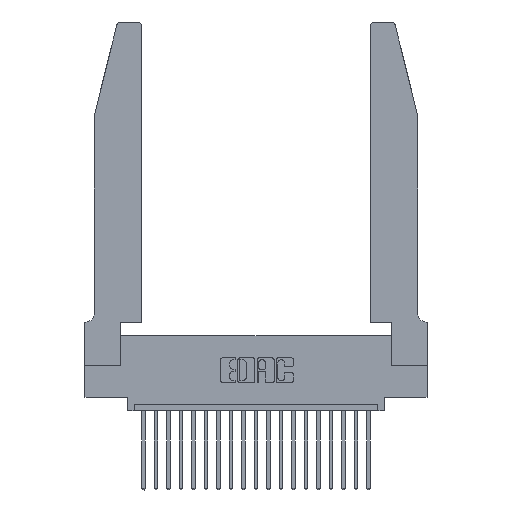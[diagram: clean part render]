
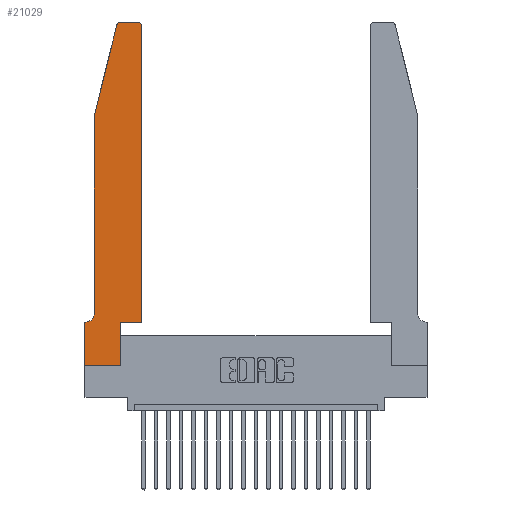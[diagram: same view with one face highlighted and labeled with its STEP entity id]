
A CAD part, top view. The second image highlights one B-rep face of the part: STEP entity #21029.
In plain terms, the highlighted planar face has unit normal (0, 0, 1).
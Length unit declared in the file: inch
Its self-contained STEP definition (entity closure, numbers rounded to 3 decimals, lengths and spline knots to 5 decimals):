
#202 = ORIENTED_EDGE ( 'NONE', *, *, #20439, .T. ) ;
#475 = FACE_OUTER_BOUND ( 'NONE', #21155, .T. ) ;
#745 = VECTOR ( 'NONE', #18518, 39.37008 ) ;
#861 = VECTOR ( 'NONE', #21753, 39.37008 ) ;
#864 = CARTESIAN_POINT ( 'NONE',  ( 0.2865, 0.35, 0.37 ) ) ;
#910 = CIRCLE ( 'NONE', #21484, 0.03 ) ;
#933 = CARTESIAN_POINT ( 'NONE',  ( 0., 0.35, 0.37 ) ) ;
#1227 = DIRECTION ( 'NONE',  ( 0., -1., 0. ) ) ;
#1330 = CARTESIAN_POINT ( 'NONE',  ( 0.2865, 0.35, 0.37 ) ) ;
#1549 = LINE ( 'NONE', #8775, #1835 ) ;
#1553 = EDGE_CURVE ( 'NONE', #18526, #16632, #6762, .T. ) ;
#1835 = VECTOR ( 'NONE', #8693, 39.37008 ) ;
#2358 = DIRECTION ( 'NONE',  ( -1., 0., 0. ) ) ;
#2425 = CIRCLE ( 'NONE', #20134, 0.07 ) ;
#2496 = DIRECTION ( 'NONE',  ( 0., 0., 1. ) ) ;
#2521 = ORIENTED_EDGE ( 'NONE', *, *, #2950, .T. ) ;
#2777 = VECTOR ( 'NONE', #1227, 39.37008 ) ;
#2950 = EDGE_CURVE ( 'NONE', #14759, #15121, #18261, .T. ) ;
#2978 = CARTESIAN_POINT ( 'NONE',  ( 0.0755, 2., 0.37 ) ) ;
#3802 = VECTOR ( 'NONE', #17745, 39.37008 ) ;
#3931 = VERTEX_POINT ( 'NONE', #5555 ) ;
#4231 = EDGE_CURVE ( 'NONE', #15005, #18241, #13648, .T. ) ;
#4685 = PLANE ( 'NONE',  #15133 ) ;
#5212 = DIRECTION ( 'NONE',  ( -1., 0., 0. ) ) ;
#5555 = CARTESIAN_POINT ( 'NONE',  ( 0.2865, 0., 0.37 ) ) ;
#5576 = CARTESIAN_POINT ( 'NONE',  ( 0.4505, 0.35, 0.37 ) ) ;
#5680 = EDGE_CURVE ( 'NONE', #15121, #8326, #12274, .T. ) ;
#6691 = AXIS2_PLACEMENT_3D ( 'NONE', #21542, #2496, #19594 ) ;
#6755 = VERTEX_POINT ( 'NONE', #10469 ) ;
#6762 = LINE ( 'NONE', #5576, #3802 ) ;
#6979 = ORIENTED_EDGE ( 'NONE', *, *, #16022, .T. ) ;
#7459 = DIRECTION ( 'NONE',  ( 0., 0., 1. ) ) ;
#7564 = LINE ( 'NONE', #1330, #10790 ) ;
#8105 = CARTESIAN_POINT ( 'NONE',  ( 0.4505, 0.35, 0.37 ) ) ;
#8278 = EDGE_CURVE ( 'NONE', #6755, #16567, #19460, .T. ) ;
#8314 = CARTESIAN_POINT ( 'NONE',  ( 0.0755, 2., 0.37 ) ) ;
#8326 = VERTEX_POINT ( 'NONE', #18783 ) ;
#8382 = DIRECTION ( 'NONE',  ( 0., 1., 0. ) ) ;
#8669 = CARTESIAN_POINT ( 'NONE',  ( 0., 0., 0.37 ) ) ;
#8693 = DIRECTION ( 'NONE',  ( -1., 0., 0. ) ) ;
#8696 = CARTESIAN_POINT ( 'NONE',  ( 0.0055, 0.42, 0.37 ) ) ;
#8775 = CARTESIAN_POINT ( 'NONE',  ( 0.2605, 2.75, 0.37 ) ) ;
#9259 = ORIENTED_EDGE ( 'NONE', *, *, #21108, .T. ) ;
#9622 = EDGE_CURVE ( 'NONE', #16632, #15005, #14655, .T. ) ;
#9852 = ORIENTED_EDGE ( 'NONE', *, *, #13249, .T. ) ;
#9885 = DIRECTION ( 'NONE',  ( 0., 0., 1. ) ) ;
#10398 = DIRECTION ( 'NONE',  ( 1., 0., 0. ) ) ;
#10469 = CARTESIAN_POINT ( 'NONE',  ( 0.0755, 2., 0.37 ) ) ;
#10790 = VECTOR ( 'NONE', #8382, 39.37008 ) ;
#11171 = CARTESIAN_POINT ( 'NONE',  ( 0., 0., 0.37 ) ) ;
#11232 = VECTOR ( 'NONE', #10398, 39.37008 ) ;
#11288 = ORIENTED_EDGE ( 'NONE', *, *, #1553, .T. ) ;
#12167 = DIRECTION ( 'NONE',  ( 0., 0., -1. ) ) ;
#12274 = LINE ( 'NONE', #11171, #14960 ) ;
#12591 = ORIENTED_EDGE ( 'NONE', *, *, #5680, .T. ) ;
#12627 = DIRECTION ( 'NONE',  ( 1., 0., 0. ) ) ;
#12697 = CARTESIAN_POINT ( 'NONE',  ( 0.284, 2.72, 0.37 ) ) ;
#13249 = EDGE_CURVE ( 'NONE', #8326, #3931, #22232, .T. ) ;
#13416 = CARTESIAN_POINT ( 'NONE',  ( 0.4505, 2.72, 0.37 ) ) ;
#13547 = ORIENTED_EDGE ( 'NONE', *, *, #4231, .T. ) ;
#13581 = CARTESIAN_POINT ( 'NONE',  ( 0.0055, 0.35, 0.37 ) ) ;
#13648 = CIRCLE ( 'NONE', #6691, 0.03 ) ;
#13654 = VERTEX_POINT ( 'NONE', #16414 ) ;
#13687 = VECTOR ( 'NONE', #2358, 39.37008 ) ;
#13944 = ORIENTED_EDGE ( 'NONE', *, *, #15004, .T. ) ;
#13973 = EDGE_CURVE ( 'NONE', #13654, #15140, #910, .T. ) ;
#14542 = CARTESIAN_POINT ( 'NONE',  ( 0.0755, 0.35, 0.37 ) ) ;
#14655 = LINE ( 'NONE', #8105, #861 ) ;
#14759 = VERTEX_POINT ( 'NONE', #13581 ) ;
#14960 = VECTOR ( 'NONE', #18667, 39.37008 ) ;
#15004 = EDGE_CURVE ( 'NONE', #3931, #18526, #7564, .T. ) ;
#15005 = VERTEX_POINT ( 'NONE', #13416 ) ;
#15121 = VERTEX_POINT ( 'NONE', #933 ) ;
#15133 = AXIS2_PLACEMENT_3D ( 'NONE', #16720, #9885, #18732 ) ;
#15140 = VERTEX_POINT ( 'NONE', #16329 ) ;
#16022 = EDGE_CURVE ( 'NONE', #18241, #13654, #1549, .T. ) ;
#16054 = CARTESIAN_POINT ( 'NONE',  ( 0.0755, 0.42, 0.37 ) ) ;
#16329 = CARTESIAN_POINT ( 'NONE',  ( 0.25487, 2.72718, 0.37 ) ) ;
#16414 = CARTESIAN_POINT ( 'NONE',  ( 0.284, 2.75, 0.37 ) ) ;
#16567 = VERTEX_POINT ( 'NONE', #16054 ) ;
#16632 = VERTEX_POINT ( 'NONE', #18365 ) ;
#16720 = CARTESIAN_POINT ( 'NONE',  ( 0., 0.35, 0.37 ) ) ;
#17298 = ORIENTED_EDGE ( 'NONE', *, *, #13973, .T. ) ;
#17745 = DIRECTION ( 'NONE',  ( 1., 0., 0. ) ) ;
#17754 = CARTESIAN_POINT ( 'NONE',  ( 0.4205, 2.75, 0.37 ) ) ;
#18241 = VERTEX_POINT ( 'NONE', #17754 ) ;
#18261 = LINE ( 'NONE', #14542, #13687 ) ;
#18365 = CARTESIAN_POINT ( 'NONE',  ( 0.4505, 0.35, 0.37 ) ) ;
#18518 = DIRECTION ( 'NONE',  ( -0.239, -0.971, 0. ) ) ;
#18526 = VERTEX_POINT ( 'NONE', #864 ) ;
#18667 = DIRECTION ( 'NONE',  ( 0., -1., 0. ) ) ;
#18732 = DIRECTION ( 'NONE',  ( 1., 0., 0. ) ) ;
#18783 = CARTESIAN_POINT ( 'NONE',  ( 0., 0., 0.37 ) ) ;
#18940 = ORIENTED_EDGE ( 'NONE', *, *, #9622, .T. ) ;
#19460 = LINE ( 'NONE', #2978, #2777 ) ;
#19594 = DIRECTION ( 'NONE',  ( 1., 0., 0. ) ) ;
#20134 = AXIS2_PLACEMENT_3D ( 'NONE', #8696, #12167, #5212 ) ;
#20439 = EDGE_CURVE ( 'NONE', #16567, #14759, #2425, .T. ) ;
#20948 = ORIENTED_EDGE ( 'NONE', *, *, #8278, .T. ) ;
#20951 = LINE ( 'NONE', #8314, #745 ) ;
#21029 = ADVANCED_FACE ( 'NONE', ( #475 ), #4685, .T. ) ;
#21108 = EDGE_CURVE ( 'NONE', #15140, #6755, #20951, .T. ) ;
#21155 = EDGE_LOOP ( 'NONE', ( #6979, #17298, #9259, #20948, #202, #2521, #12591, #9852, #13944, #11288, #18940, #13547 ) ) ;
#21484 = AXIS2_PLACEMENT_3D ( 'NONE', #12697, #7459, #12627 ) ;
#21542 = CARTESIAN_POINT ( 'NONE',  ( 0.4205, 2.72, 0.37 ) ) ;
#21753 = DIRECTION ( 'NONE',  ( 0., 1., 0. ) ) ;
#22232 = LINE ( 'NONE', #8669, #11232 ) ;
